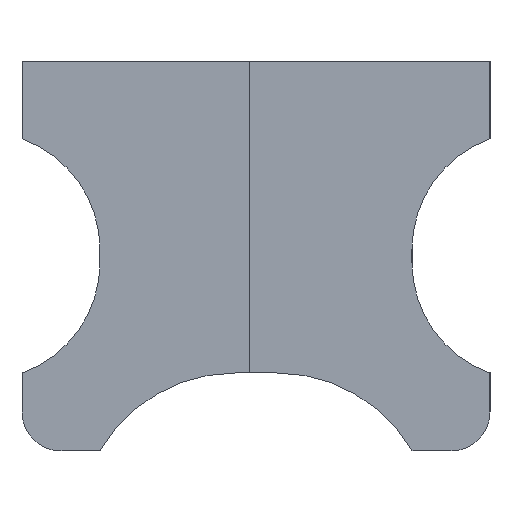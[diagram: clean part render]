
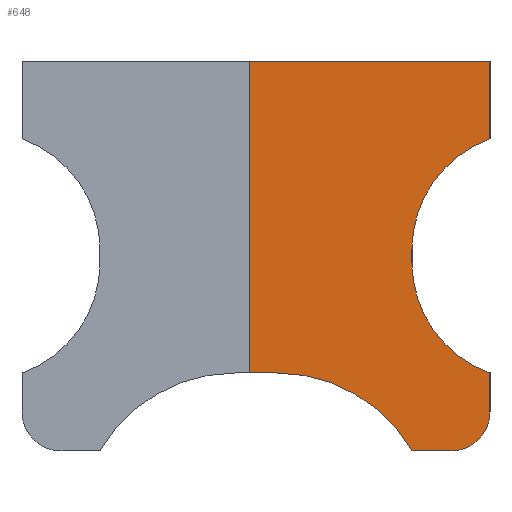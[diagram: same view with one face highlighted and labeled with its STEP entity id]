
A CAD part, left-side view. The second image highlights one B-rep face of the part: STEP entity #648.
In plain terms, the highlighted planar face has unit normal (-1, 0, 0).
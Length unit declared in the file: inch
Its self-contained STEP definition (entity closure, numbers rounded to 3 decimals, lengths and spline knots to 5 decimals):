
#9 = CARTESIAN_POINT ( 'NONE',  ( -1.9472, -0.57034, 0. ) ) ;
#16 = DIRECTION ( 'NONE',  ( 0., 0., 1. ) ) ;
#18 = VERTEX_POINT ( 'NONE', #51 ) ;
#19 = VERTEX_POINT ( 'NONE', #190 ) ;
#26 = CARTESIAN_POINT ( 'NONE',  ( -1.9472, -0.60971, 0.1018 ) ) ;
#28 = DIRECTION ( 'NONE',  ( 0., 1., 0. ) ) ;
#33 = VECTOR ( 'NONE', #635, 39.37008 ) ;
#39 = VERTEX_POINT ( 'NONE', #129 ) ;
#51 = CARTESIAN_POINT ( 'NONE',  ( -1.9472, -0.55065, 0.1018 ) ) ;
#52 = VECTOR ( 'NONE', #153, 39.37008 ) ;
#68 = CIRCLE ( 'NONE', #255, 0.01969 ) ;
#82 = DIRECTION ( 'NONE',  ( 0., -1., 0. ) ) ;
#92 = DIRECTION ( 'NONE',  ( -1., 0., 0. ) ) ;
#105 = FACE_OUTER_BOUND ( 'NONE', #350, .T. ) ;
#126 = VERTEX_POINT ( 'NONE', #9 ) ;
#129 = CARTESIAN_POINT ( 'NONE',  ( -1.9472, -0.46882, 0.03937 ) ) ;
#130 = CARTESIAN_POINT ( 'NONE',  ( -1.9472, -0.59002, 0.15748 ) ) ;
#134 = ORIENTED_EDGE ( 'NONE', *, *, #531, .T. ) ;
#135 = DIRECTION ( 'NONE',  ( 1., 0., 0. ) ) ;
#142 = CARTESIAN_POINT ( 'NONE',  ( -1.9472, 0., 0.03937 ) ) ;
#146 = DIRECTION ( 'NONE',  ( 0., -1., 0. ) ) ;
#153 = DIRECTION ( 'NONE',  ( 0., 0., 1. ) ) ;
#164 = LINE ( 'NONE', #621, #326 ) ;
#190 = CARTESIAN_POINT ( 'NONE',  ( -1.9472, -0.46882, 0.19685 ) ) ;
#199 = LINE ( 'NONE', #421, #358 ) ;
#203 = ORIENTED_EDGE ( 'NONE', *, *, #526, .T. ) ;
#208 = AXIS2_PLACEMENT_3D ( 'NONE', #508, #92, #583 ) ;
#224 = VERTEX_POINT ( 'NONE', #473 ) ;
#238 = AXIS2_PLACEMENT_3D ( 'NONE', #26, #490, #82 ) ;
#240 = VECTOR ( 'NONE', #28, 39.37008 ) ;
#244 = AXIS2_PLACEMENT_3D ( 'NONE', #488, #135, #683 ) ;
#253 = ORIENTED_EDGE ( 'NONE', *, *, #514, .T. ) ;
#255 = AXIS2_PLACEMENT_3D ( 'NONE', #288, #747, #356 ) ;
#262 = LINE ( 'NONE', #142, #240 ) ;
#266 = AXIS2_PLACEMENT_3D ( 'NONE', #286, #745, #352 ) ;
#278 = VERTEX_POINT ( 'NONE', #671 ) ;
#281 = DIRECTION ( 'NONE',  ( 0., 0., 1. ) ) ;
#286 = CARTESIAN_POINT ( 'NONE',  ( -1.9472, -0.48246, -0.03937 ) ) ;
#288 = CARTESIAN_POINT ( 'NONE',  ( -1.9472, -0.57034, 0.01969 ) ) ;
#321 = ORIENTED_EDGE ( 'NONE', *, *, #532, .T. ) ;
#326 = VECTOR ( 'NONE', #16, 39.37008 ) ;
#347 = CARTESIAN_POINT ( 'NONE',  ( -1.9472, 0., 0.19685 ) ) ;
#350 = EDGE_LOOP ( 'NONE', ( #587, #579, #378, #253, #724, #628, #203, #134, #321, #764, #695 ) ) ;
#352 = DIRECTION ( 'NONE',  ( 0., -1., 0. ) ) ;
#356 = DIRECTION ( 'NONE',  ( 0., -1., 0. ) ) ;
#358 = VECTOR ( 'NONE', #281, 39.37008 ) ;
#378 = ORIENTED_EDGE ( 'NONE', *, *, #509, .F. ) ;
#384 = CIRCLE ( 'NONE', #238, 0.05906 ) ;
#389 = VERTEX_POINT ( 'NONE', #714 ) ;
#405 = CIRCLE ( 'NONE', #244, 0.05906 ) ;
#421 = CARTESIAN_POINT ( 'NONE',  ( -1.9472, -0.59002, 0.19685 ) ) ;
#422 = VERTEX_POINT ( 'NONE', #664 ) ;
#423 = DIRECTION ( 'NONE',  ( 0., -1., 0. ) ) ;
#445 = LINE ( 'NONE', #347, #611 ) ;
#451 = VERTEX_POINT ( 'NONE', #130 ) ;
#456 = EDGE_CURVE ( 'NONE', #39, #19, #164, .T. ) ;
#473 = CARTESIAN_POINT ( 'NONE',  ( -1.9472, -0.55065, 0.09505 ) ) ;
#488 = CARTESIAN_POINT ( 'NONE',  ( -1.9472, -0.60971, 0.09505 ) ) ;
#490 = DIRECTION ( 'NONE',  ( 1., 0., 0. ) ) ;
#505 = EDGE_CURVE ( 'NONE', #19, #511, #445, .T. ) ;
#508 = CARTESIAN_POINT ( 'NONE',  ( -1.9472, -0.46882, -1.26417 ) ) ;
#509 = EDGE_CURVE ( 'NONE', #389, #39, #262, .T. ) ;
#511 = VERTEX_POINT ( 'NONE', #790 ) ;
#514 = EDGE_CURVE ( 'NONE', #389, #422, #746, .T. ) ;
#516 = EDGE_CURVE ( 'NONE', #422, #126, #761, .T. ) ;
#521 = EDGE_CURVE ( 'NONE', #278, #126, #68, .T. ) ;
#526 = EDGE_CURVE ( 'NONE', #278, #657, #573, .T. ) ;
#531 = EDGE_CURVE ( 'NONE', #657, #224, #405, .T. ) ;
#532 = EDGE_CURVE ( 'NONE', #224, #18, #727, .T. ) ;
#537 = EDGE_CURVE ( 'NONE', #18, #451, #384, .T. ) ;
#542 = EDGE_CURVE ( 'NONE', #451, #511, #199, .T. ) ;
#573 = LINE ( 'NONE', #574, #52 ) ;
#574 = CARTESIAN_POINT ( 'NONE',  ( -1.9472, -0.59002, 0.19685 ) ) ;
#579 = ORIENTED_EDGE ( 'NONE', *, *, #456, .F. ) ;
#583 = DIRECTION ( 'NONE',  ( 0., -1., 0. ) ) ;
#587 = ORIENTED_EDGE ( 'NONE', *, *, #505, .F. ) ;
#592 = VECTOR ( 'NONE', #146, 39.37008 ) ;
#611 = VECTOR ( 'NONE', #423, 39.37008 ) ;
#621 = CARTESIAN_POINT ( 'NONE',  ( -1.9472, -0.46882, -1.26417 ) ) ;
#628 = ORIENTED_EDGE ( 'NONE', *, *, #521, .F. ) ;
#631 = CARTESIAN_POINT ( 'NONE',  ( -1.9472, -0.55065, 0.09843 ) ) ;
#635 = DIRECTION ( 'NONE',  ( 0., 0., 1. ) ) ;
#648 = ADVANCED_FACE ( 'NONE', ( #105 ), #754, .T. ) ;
#657 = VERTEX_POINT ( 'NONE', #700 ) ;
#664 = CARTESIAN_POINT ( 'NONE',  ( -1.9472, -0.55065, 0. ) ) ;
#671 = CARTESIAN_POINT ( 'NONE',  ( -1.9472, -0.59002, 0.01969 ) ) ;
#683 = DIRECTION ( 'NONE',  ( 0., -1., 0. ) ) ;
#688 = CARTESIAN_POINT ( 'NONE',  ( -1.9472, 0., 0. ) ) ;
#695 = ORIENTED_EDGE ( 'NONE', *, *, #542, .T. ) ;
#700 = CARTESIAN_POINT ( 'NONE',  ( -1.9472, -0.59002, 0.03937 ) ) ;
#714 = CARTESIAN_POINT ( 'NONE',  ( -1.9472, -0.48246, 0.03937 ) ) ;
#724 = ORIENTED_EDGE ( 'NONE', *, *, #516, .T. ) ;
#727 = LINE ( 'NONE', #631, #33 ) ;
#745 = DIRECTION ( 'NONE',  ( 1., 0., 0. ) ) ;
#746 = CIRCLE ( 'NONE', #266, 0.07874 ) ;
#747 = DIRECTION ( 'NONE',  ( 1., 0., 0. ) ) ;
#754 = PLANE ( 'NONE',  #208 ) ;
#761 = LINE ( 'NONE', #688, #592 ) ;
#764 = ORIENTED_EDGE ( 'NONE', *, *, #537, .T. ) ;
#790 = CARTESIAN_POINT ( 'NONE',  ( -1.9472, -0.59002, 0.19685 ) ) ;
